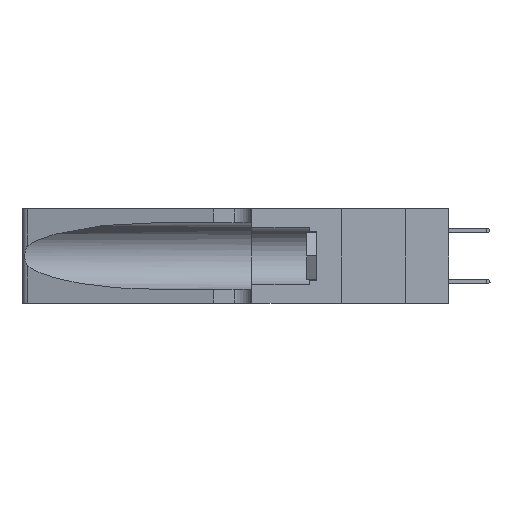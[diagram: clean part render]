
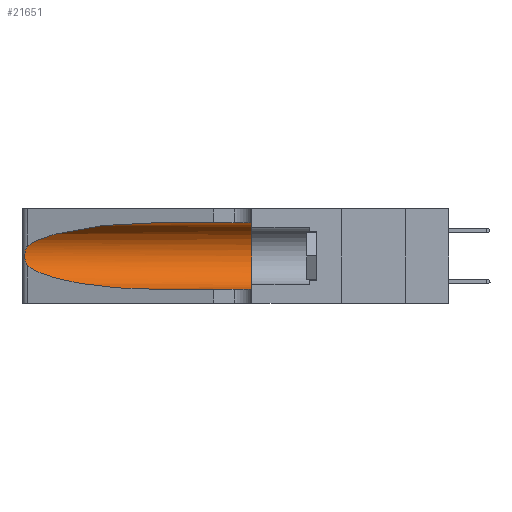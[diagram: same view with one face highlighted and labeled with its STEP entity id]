
A CAD part, left-side view. The second image highlights one B-rep face of the part: STEP entity #21651.
In plain terms, the highlighted cylindrical face has radius 3.308 mm (diameter 6.617 mm), a partial arc.
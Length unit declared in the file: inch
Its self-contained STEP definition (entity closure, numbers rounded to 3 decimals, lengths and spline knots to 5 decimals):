
#304 = CARTESIAN_POINT ( 'NONE',  ( 0.25487, 1.22718, 0.22369 ) ) ;
#365 = EDGE_CURVE ( 'NONE', #41613, #34900, #45155, .T. ) ;
#376 = CARTESIAN_POINT ( 'NONE',  ( 0.18966, 0.96281, 0.31525 ) ) ;
#1918 = DIRECTION ( 'NONE',  ( 0., -1., 0. ) ) ;
#2835 = CARTESIAN_POINT ( 'NONE',  ( 0.26075, 1.23896, 0.19203 ) ) ;
#3610 = CARTESIAN_POINT ( 'NONE',  ( 0.1305, 0.35, 0.05475 ) ) ;
#3617 = DIRECTION ( 'NONE',  ( 0., 0., -1. ) ) ;
#3832 = DIRECTION ( 'NONE',  ( 0., 0., 1. ) ) ;
#4243 = CARTESIAN_POINT ( 'NONE',  ( 0.25487, 1.22718, 0.22369 ) ) ;
#5449 = CARTESIAN_POINT ( 'NONE',  ( 0.1305, 0.72297, 0.05475 ) ) ;
#6673 = CARTESIAN_POINT ( 'NONE',  ( 0.26017, 1.23833, 0.17102 ) ) ;
#8620 = CARTESIAN_POINT ( 'NONE',  ( 0.1305, 0.72297, 0.31525 ) ) ;
#9768 = CYLINDRICAL_SURFACE ( 'NONE', #10006, 0.13025 ) ;
#9779 = CARTESIAN_POINT ( 'NONE',  ( 0.18966, 0.96281, 0.05475 ) ) ;
#10006 = AXIS2_PLACEMENT_3D ( 'NONE', #26436, #41395, #3617 ) ;
#10391 = CARTESIAN_POINT ( 'NONE',  ( 0.25555, 1.22994, 0.2215 ) ) ;
#10554 = CARTESIAN_POINT ( 'NONE',  ( 0.25789, 1.23486, 0.15765 ) ) ;
#12148 = CARTESIAN_POINT ( 'NONE',  ( 0.1305, 0.35, 0.31525 ) ) ;
#13169 = ORIENTED_EDGE ( 'NONE', *, *, #46640, .F. ) ;
#13452 = CARTESIAN_POINT ( 'NONE',  ( 0.1305, 0.35, 0.185 ) ) ;
#13630 = CARTESIAN_POINT ( 'NONE',  ( 0.1305, 0.72297, 0.05475 ) ) ;
#14404 = CARTESIAN_POINT ( 'NONE',  ( 0.25555, 1.22993, 0.14849 ) ) ;
#14834 = VERTEX_POINT ( 'NONE', #8620 ) ;
#15293 = B_SPLINE_CURVE_WITH_KNOTS ( 'NONE', 3,
 ( #40624, #10391, #44373, #21832, #48110, #25625, #2835, #29438, #6673, #33264, #10554, #37041, #14404, #40786 ),
 .UNSPECIFIED., .F., .F.,
 ( 4, 2, 2, 2, 2, 2, 4 ),
 ( 0., 0.00027, 0.00053, 0.00107, 0.0016, 0.00187, 0.00214 ),
 .UNSPECIFIED. ) ;
#15423 = ORIENTED_EDGE ( 'NONE', *, *, #24203, .T. ) ;
#16575 = VERTEX_POINT ( 'NONE', #3610 ) ;
#20376 = VERTEX_POINT ( 'NONE', #12148 ) ;
#20449 = EDGE_LOOP ( 'NONE', ( #15423, #35523, #31489, #44959, #13169, #36847 ) ) ;
#21651 = ADVANCED_FACE ( 'NONE', ( #29940 ), #9768, .F. ) ;
#21766 = EDGE_CURVE ( 'NONE', #14834, #20376, #45167, .T. ) ;
#21832 = CARTESIAN_POINT ( 'NONE',  ( 0.25787, 1.23484, 0.2124 ) ) ;
#23289 = CARTESIAN_POINT ( 'NONE',  ( 0.1305, 1.61858, 0.31525 ) ) ;
#24203 = EDGE_CURVE ( 'NONE', #14834, #46718, #32889, .T. ) ;
#25625 = CARTESIAN_POINT ( 'NONE',  ( 0.26018, 1.23835, 0.19895 ) ) ;
#26436 = CARTESIAN_POINT ( 'NONE',  ( 0.1305, 1.61858, 0.185 ) ) ;
#26647 = DIRECTION ( 'NONE',  ( 0., 1., 0. ) ) ;
#27040 = CARTESIAN_POINT ( 'NONE',  ( 0.2373, 1.15595, 0.28018 ) ) ;
#27556 = VECTOR ( 'NONE', #30898, 39.37008 ) ;
#28549 = CARTESIAN_POINT ( 'NONE',  ( 0.1305, 1.61858, 0.05475 ) ) ;
#29197 = CIRCLE ( 'NONE', #36697, 0.13025 ) ;
#29438 = CARTESIAN_POINT ( 'NONE',  ( 0.26075, 1.23896, 0.178 ) ) ;
#29940 = FACE_OUTER_BOUND ( 'NONE', #20449, .T. ) ;
#30361 = EDGE_CURVE ( 'NONE', #46718, #41613, #15293, .T. ) ;
#30898 = DIRECTION ( 'NONE',  ( 0., -1., 0. ) ) ;
#31489 = ORIENTED_EDGE ( 'NONE', *, *, #365, .T. ) ;
#32502 = CARTESIAN_POINT ( 'NONE',  ( 0.2373, 1.15595, 0.08982 ) ) ;
#32889 =( BOUNDED_CURVE ( )  B_SPLINE_CURVE ( 3, ( #45756, #376, #27040, #4243 ),
 .UNSPECIFIED., .F., .F. ) 
 B_SPLINE_CURVE_WITH_KNOTS ( ( 4, 4 ),
 ( 1.5708, 2.84003 ),
 .UNSPECIFIED. ) 
 CURVE ( )  GEOMETRIC_REPRESENTATION_ITEM ( )  RATIONAL_B_SPLINE_CURVE ( ( 1., 0.87, 0.87, 1. ) ) 
 REPRESENTATION_ITEM ( '' )  );
#33264 = CARTESIAN_POINT ( 'NONE',  ( 0.25856, 1.23593, 0.16098 ) ) ;
#34900 = VERTEX_POINT ( 'NONE', #5449 ) ;
#35523 = ORIENTED_EDGE ( 'NONE', *, *, #30361, .T. ) ;
#36279 = CARTESIAN_POINT ( 'NONE',  ( 0.25487, 1.22718, 0.14631 ) ) ;
#36697 = AXIS2_PLACEMENT_3D ( 'NONE', #13452, #26647, #3832 ) ;
#36847 = ORIENTED_EDGE ( 'NONE', *, *, #21766, .F. ) ;
#37041 = CARTESIAN_POINT ( 'NONE',  ( 0.25639, 1.23186, 0.15144 ) ) ;
#39347 = LINE ( 'NONE', #28549, #44564 ) ;
#40624 = CARTESIAN_POINT ( 'NONE',  ( 0.25487, 1.22718, 0.22369 ) ) ;
#40786 = CARTESIAN_POINT ( 'NONE',  ( 0.25487, 1.22718, 0.14631 ) ) ;
#41395 = DIRECTION ( 'NONE',  ( 0., -1., 0. ) ) ;
#41613 = VERTEX_POINT ( 'NONE', #43951 ) ;
#43951 = CARTESIAN_POINT ( 'NONE',  ( 0.25487, 1.22718, 0.14631 ) ) ;
#44373 = CARTESIAN_POINT ( 'NONE',  ( 0.25639, 1.23184, 0.21858 ) ) ;
#44564 = VECTOR ( 'NONE', #1918, 39.37008 ) ;
#44959 = ORIENTED_EDGE ( 'NONE', *, *, #45759, .T. ) ;
#45155 =( BOUNDED_CURVE ( )  B_SPLINE_CURVE ( 3, ( #36279, #32502, #9779, #13630 ),
 .UNSPECIFIED., .F., .F. ) 
 B_SPLINE_CURVE_WITH_KNOTS ( ( 4, 4 ),
 ( 3.44316, 4.71239 ),
 .UNSPECIFIED. ) 
 CURVE ( )  GEOMETRIC_REPRESENTATION_ITEM ( )  RATIONAL_B_SPLINE_CURVE ( ( 1., 0.87, 0.87, 1. ) ) 
 REPRESENTATION_ITEM ( '' )  );
#45167 = LINE ( 'NONE', #23289, #27556 ) ;
#45756 = CARTESIAN_POINT ( 'NONE',  ( 0.1305, 0.72297, 0.31525 ) ) ;
#45759 = EDGE_CURVE ( 'NONE', #34900, #16575, #39347, .T. ) ;
#46640 = EDGE_CURVE ( 'NONE', #20376, #16575, #29197, .T. ) ;
#46718 = VERTEX_POINT ( 'NONE', #304 ) ;
#48110 = CARTESIAN_POINT ( 'NONE',  ( 0.25854, 1.2359, 0.20912 ) ) ;
